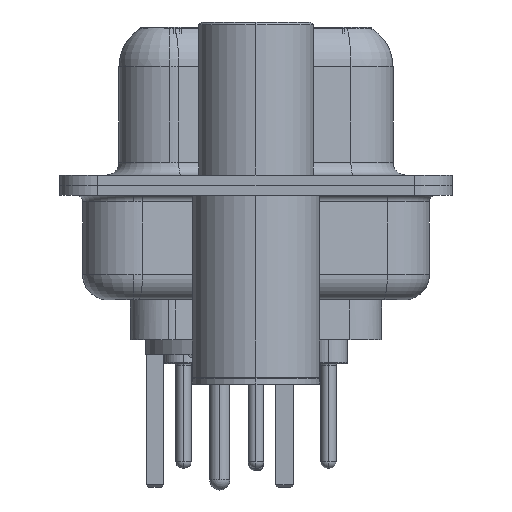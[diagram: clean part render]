
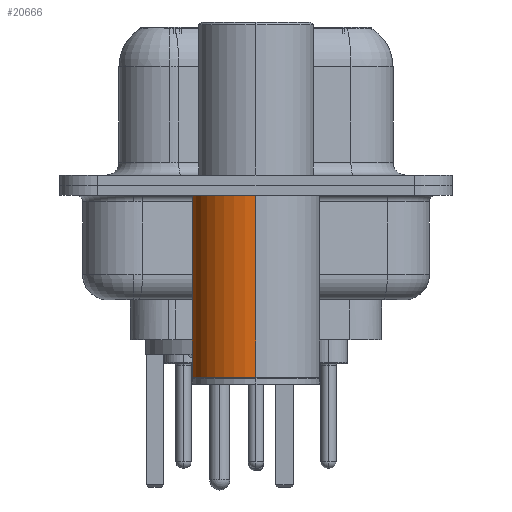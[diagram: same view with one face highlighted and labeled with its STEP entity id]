
A CAD part, left-side view. The second image highlights one B-rep face of the part: STEP entity #20666.
In plain terms, the highlighted cylindrical face has radius 2.5 mm (diameter 5 mm), a partial arc.
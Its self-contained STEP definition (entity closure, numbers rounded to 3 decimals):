
#1222 = CARTESIAN_POINT ( 'NONE',  ( -2.5, 0., 0.581 ) ) ;
#3170 = VECTOR ( 'NONE', #12252, 1000. ) ;
#3346 = ORIENTED_EDGE ( 'NONE', *, *, #19814, .T. ) ;
#4042 = DIRECTION ( 'NONE',  ( 1., 0., 0. ) ) ;
#5277 = LINE ( 'NONE', #1222, #24759 ) ;
#5986 = ORIENTED_EDGE ( 'NONE', *, *, #8258, .F. ) ;
#8258 = EDGE_CURVE ( 'NONE', #35719, #19198, #13198, .T. ) ;
#9011 = CARTESIAN_POINT ( 'NONE',  ( 0., 0., -0.4 ) ) ;
#10396 = VERTEX_POINT ( 'NONE', #14554 ) ;
#11571 = ORIENTED_EDGE ( 'NONE', *, *, #17854, .F. ) ;
#11715 = VERTEX_POINT ( 'NONE', #15664 ) ;
#12252 = DIRECTION ( 'NONE',  ( 0., 0., 1. ) ) ;
#13198 = CIRCLE ( 'NONE', #24244, 2.5 ) ;
#13664 = EDGE_LOOP ( 'NONE', ( #3346, #29714, #5986, #11571 ) ) ;
#14554 = CARTESIAN_POINT ( 'NONE',  ( -2.5, 0., -7.525 ) ) ;
#15189 = DIRECTION ( 'NONE',  ( 1., 0., 0. ) ) ;
#15664 = CARTESIAN_POINT ( 'NONE',  ( 2.5, 0., -7.525 ) ) ;
#17730 = CARTESIAN_POINT ( 'NONE',  ( 0., 0., 0.581 ) ) ;
#17853 = CIRCLE ( 'NONE', #20501, 2.5 ) ;
#17854 = EDGE_CURVE ( 'NONE', #11715, #35719, #19643, .T. ) ;
#18535 = DIRECTION ( 'NONE',  ( 1., 0., 0. ) ) ;
#19128 = CARTESIAN_POINT ( 'NONE',  ( 0., 0., -7.525 ) ) ;
#19198 = VERTEX_POINT ( 'NONE', #32059 ) ;
#19302 = CARTESIAN_POINT ( 'NONE',  ( 2.5, 0., -0.4 ) ) ;
#19643 = LINE ( 'NONE', #34129, #3170 ) ;
#19814 = EDGE_CURVE ( 'NONE', #11715, #10396, #17853, .T. ) ;
#20501 = AXIS2_PLACEMENT_3D ( 'NONE', #19128, #35075, #18535 ) ;
#20666 = ADVANCED_FACE ( 'NONE', ( #22098 ), #30712, .T. ) ;
#21456 = AXIS2_PLACEMENT_3D ( 'NONE', #17730, #28476, #15189 ) ;
#22098 = FACE_OUTER_BOUND ( 'NONE', #13664, .T. ) ;
#24244 = AXIS2_PLACEMENT_3D ( 'NONE', #9011, #31350, #4042 ) ;
#24759 = VECTOR ( 'NONE', #25943, 1000. ) ;
#25943 = DIRECTION ( 'NONE',  ( 0., 0., 1. ) ) ;
#28476 = DIRECTION ( 'NONE',  ( 0., 0., 1. ) ) ;
#29714 = ORIENTED_EDGE ( 'NONE', *, *, #31441, .T. ) ;
#30712 = CYLINDRICAL_SURFACE ( 'NONE', #21456, 2.5 ) ;
#31350 = DIRECTION ( 'NONE',  ( 0., 0., 1. ) ) ;
#31441 = EDGE_CURVE ( 'NONE', #10396, #19198, #5277, .T. ) ;
#32059 = CARTESIAN_POINT ( 'NONE',  ( -2.5, 0., -0.4 ) ) ;
#34129 = CARTESIAN_POINT ( 'NONE',  ( 2.5, 0., 0.581 ) ) ;
#35075 = DIRECTION ( 'NONE',  ( 0., 0., 1. ) ) ;
#35719 = VERTEX_POINT ( 'NONE', #19302 ) ;
